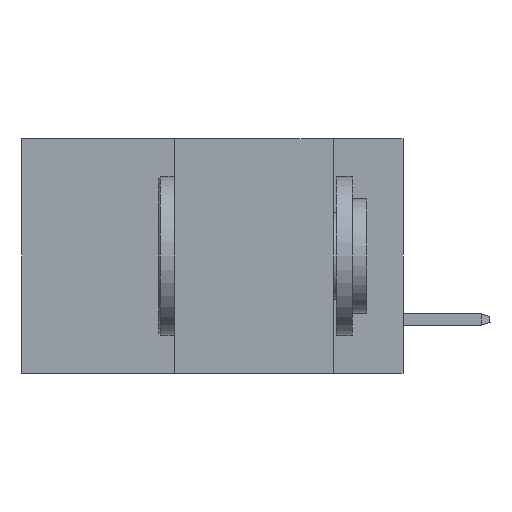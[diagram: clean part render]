
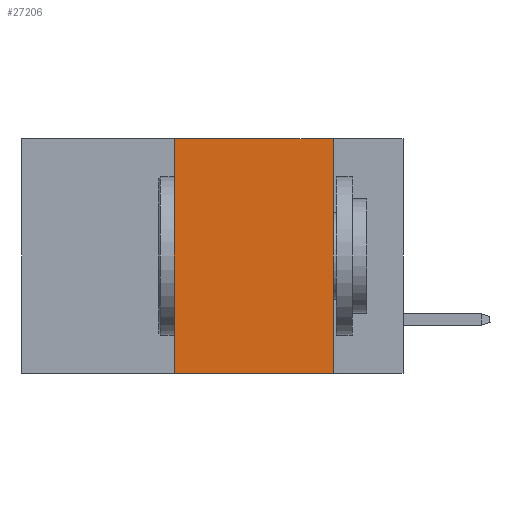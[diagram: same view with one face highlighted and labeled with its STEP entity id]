
A CAD part, left-side view. The second image highlights one B-rep face of the part: STEP entity #27206.
In plain terms, the highlighted planar face has unit normal (-1, 0, 0).
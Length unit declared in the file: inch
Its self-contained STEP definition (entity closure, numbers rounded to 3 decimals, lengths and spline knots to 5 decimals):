
#349 = CARTESIAN_POINT ( 'NONE',  ( 0., 0.11, -0.37 ) ) ;
#7356 = DIRECTION ( 'NONE',  ( 0., -1., 0. ) ) ;
#8322 = ORIENTED_EDGE ( 'NONE', *, *, #24665, .F. ) ;
#9368 = EDGE_CURVE ( 'NONE', #41507, #13762, #19507, .T. ) ;
#13762 = VERTEX_POINT ( 'NONE', #349 ) ;
#13857 = CARTESIAN_POINT ( 'NONE',  ( 0., 0.11, 0. ) ) ;
#14032 = ORIENTED_EDGE ( 'NONE', *, *, #23563, .F. ) ;
#14139 = VERTEX_POINT ( 'NONE', #22231 ) ;
#14998 = CARTESIAN_POINT ( 'NONE',  ( 0., 0.36, 0. ) ) ;
#15693 = ORIENTED_EDGE ( 'NONE', *, *, #39422, .F. ) ;
#17251 = CARTESIAN_POINT ( 'NONE',  ( 0., 0.6, 0. ) ) ;
#17683 = ORIENTED_EDGE ( 'NONE', *, *, #9368, .T. ) ;
#19507 = LINE ( 'NONE', #35091, #41734 ) ;
#22231 = CARTESIAN_POINT ( 'NONE',  ( 0., 0.11, 0. ) ) ;
#23563 = EDGE_CURVE ( 'NONE', #45802, #14139, #31825, .T. ) ;
#24665 = EDGE_CURVE ( 'NONE', #41507, #45802, #49906, .T. ) ;
#27206 = ADVANCED_FACE ( 'NONE', ( #36895 ), #29014, .F. ) ;
#28501 = DIRECTION ( 'NONE',  ( 1., 0., 0. ) ) ;
#29014 = PLANE ( 'NONE',  #29243 ) ;
#29243 = AXIS2_PLACEMENT_3D ( 'NONE', #17251, #28501, #47614 ) ;
#30574 = DIRECTION ( 'NONE',  ( 0., 0., 1. ) ) ;
#31511 = DIRECTION ( 'NONE',  ( 0., -1., 0. ) ) ;
#31825 = LINE ( 'NONE', #42284, #42811 ) ;
#32724 = EDGE_LOOP ( 'NONE', ( #15693, #14032, #8322, #17683 ) ) ;
#35091 = CARTESIAN_POINT ( 'NONE',  ( 0., 0.6, -0.37 ) ) ;
#36895 = FACE_OUTER_BOUND ( 'NONE', #32724, .T. ) ;
#37345 = DIRECTION ( 'NONE',  ( 0., 0., -1. ) ) ;
#39422 = EDGE_CURVE ( 'NONE', #14139, #13762, #40910, .T. ) ;
#39624 = VECTOR ( 'NONE', #30574, 39.37008 ) ;
#40465 = CARTESIAN_POINT ( 'NONE',  ( 0., 0.36, -0.37 ) ) ;
#40910 = LINE ( 'NONE', #13857, #49461 ) ;
#41507 = VERTEX_POINT ( 'NONE', #40465 ) ;
#41734 = VECTOR ( 'NONE', #31511, 39.37008 ) ;
#42284 = CARTESIAN_POINT ( 'NONE',  ( 0., 0.6, 0. ) ) ;
#42811 = VECTOR ( 'NONE', #7356, 39.37008 ) ;
#44433 = CARTESIAN_POINT ( 'NONE',  ( 0., 0.36, 0. ) ) ;
#45802 = VERTEX_POINT ( 'NONE', #44433 ) ;
#47614 = DIRECTION ( 'NONE',  ( 0., 0., -1. ) ) ;
#49461 = VECTOR ( 'NONE', #37345, 39.37008 ) ;
#49906 = LINE ( 'NONE', #14998, #39624 ) ;
